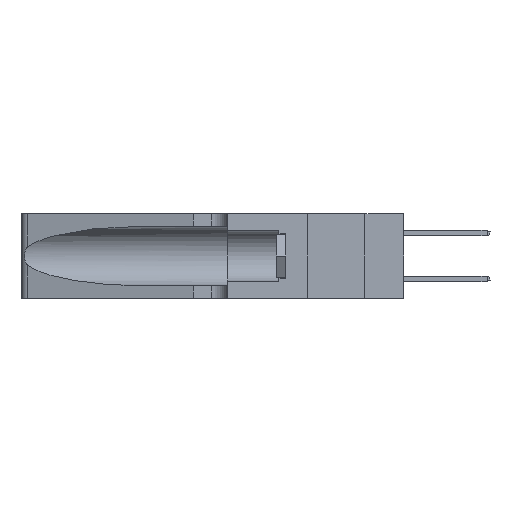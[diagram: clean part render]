
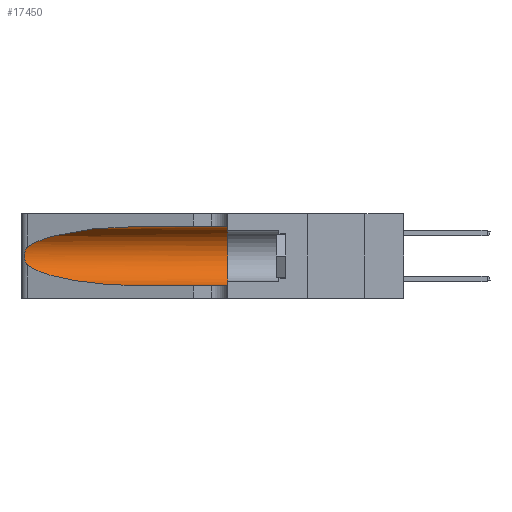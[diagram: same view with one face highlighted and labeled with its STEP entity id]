
A CAD part, left-side view. The second image highlights one B-rep face of the part: STEP entity #17450.
In plain terms, the highlighted cylindrical face has radius 3.308 mm (diameter 6.617 mm), a partial arc.
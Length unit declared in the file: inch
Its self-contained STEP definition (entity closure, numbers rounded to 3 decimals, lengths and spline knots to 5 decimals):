
#87 = CARTESIAN_POINT ( 'NONE',  ( 0.18966, 0.96281, 0.05475 ) ) ;
#588 = EDGE_CURVE ( 'NONE', #19616, #23437, #5162, .T. ) ;
#668 = CARTESIAN_POINT ( 'NONE',  ( 0.26075, 1.23896, 0.19203 ) ) ;
#1308 = CARTESIAN_POINT ( 'NONE',  ( 0.25639, 1.23186, 0.15144 ) ) ;
#2458 = CARTESIAN_POINT ( 'NONE',  ( 0.1305, 1.61858, 0.31525 ) ) ;
#2461 =( BOUNDED_CURVE ( )  B_SPLINE_CURVE ( 3, ( #14594, #11994, #22267, #20151 ),
 .UNSPECIFIED., .F., .T. ) 
 B_SPLINE_CURVE_WITH_KNOTS ( ( 4, 4 ),
 ( 1.5708, 2.84003 ),
 .UNSPECIFIED. ) 
 CURVE ( )  GEOMETRIC_REPRESENTATION_ITEM ( )  RATIONAL_B_SPLINE_CURVE ( ( 1., 0.87, 0.87, 1. ) ) 
 REPRESENTATION_ITEM ( '' )  );
#3308 = EDGE_CURVE ( 'NONE', #19616, #25562, #2461, .T. ) ;
#3708 = CARTESIAN_POINT ( 'NONE',  ( 0.1305, 0.72297, 0.05475 ) ) ;
#3767 = CARTESIAN_POINT ( 'NONE',  ( 0.25487, 1.22718, 0.22369 ) ) ;
#4150 = CARTESIAN_POINT ( 'NONE',  ( 0.1305, 0.35, 0.31525 ) ) ;
#5162 = LINE ( 'NONE', #2458, #22549 ) ;
#5173 = CARTESIAN_POINT ( 'NONE',  ( 0.25789, 1.23486, 0.15765 ) ) ;
#5747 = CARTESIAN_POINT ( 'NONE',  ( 0.25487, 1.22718, 0.14631 ) ) ;
#5825 = CARTESIAN_POINT ( 'NONE',  ( 0.26018, 1.23835, 0.19895 ) ) ;
#6298 = ORIENTED_EDGE ( 'NONE', *, *, #21303, .F. ) ;
#6315 = CARTESIAN_POINT ( 'NONE',  ( 0.25487, 1.22718, 0.22369 ) ) ;
#7749 = CARTESIAN_POINT ( 'NONE',  ( 0.1305, 1.61858, 0.185 ) ) ;
#7770 = CARTESIAN_POINT ( 'NONE',  ( 0.25639, 1.23184, 0.21858 ) ) ;
#8176 = EDGE_LOOP ( 'NONE', ( #15291, #21233, #22912, #13807, #6298, #23197 ) ) ;
#8428 = DIRECTION ( 'NONE',  ( 0., -1., 0. ) ) ;
#8626 = CARTESIAN_POINT ( 'NONE',  ( 0.26075, 1.23896, 0.178 ) ) ;
#9104 = CARTESIAN_POINT ( 'NONE',  ( 0.25854, 1.2359, 0.20912 ) ) ;
#9797 = VERTEX_POINT ( 'NONE', #15335 ) ;
#9818 = CARTESIAN_POINT ( 'NONE',  ( 0.2373, 1.15595, 0.08982 ) ) ;
#9870 = AXIS2_PLACEMENT_3D ( 'NONE', #19669, #17270, #13297 ) ;
#9951 = CIRCLE ( 'NONE', #9870, 0.13025 ) ;
#11065 = CARTESIAN_POINT ( 'NONE',  ( 0.25555, 1.22994, 0.2215 ) ) ;
#11994 = CARTESIAN_POINT ( 'NONE',  ( 0.18966, 0.96281, 0.31525 ) ) ;
#12639 = VERTEX_POINT ( 'NONE', #22845 ) ;
#13208 = CARTESIAN_POINT ( 'NONE',  ( 0.25856, 1.23593, 0.16098 ) ) ;
#13297 = DIRECTION ( 'NONE',  ( 0., 0., 1. ) ) ;
#13752 = DIRECTION ( 'NONE',  ( 0., 0., -1. ) ) ;
#13782 = CARTESIAN_POINT ( 'NONE',  ( 0.25787, 1.23484, 0.2124 ) ) ;
#13807 = ORIENTED_EDGE ( 'NONE', *, *, #19516, .T. ) ;
#13856 = VECTOR ( 'NONE', #8428, 39.37008 ) ;
#14523 = EDGE_CURVE ( 'NONE', #25562, #9797, #21310, .T. ) ;
#14594 = CARTESIAN_POINT ( 'NONE',  ( 0.1305, 0.72297, 0.31525 ) ) ;
#15291 = ORIENTED_EDGE ( 'NONE', *, *, #3308, .T. ) ;
#15335 = CARTESIAN_POINT ( 'NONE',  ( 0.25487, 1.22718, 0.14631 ) ) ;
#15519 = CARTESIAN_POINT ( 'NONE',  ( 0.25487, 1.22718, 0.14631 ) ) ;
#17270 = DIRECTION ( 'NONE',  ( 0., 1., 0. ) ) ;
#17450 = ADVANCED_FACE ( 'NONE', ( #18200 ), #18856, .F. ) ;
#18200 = FACE_OUTER_BOUND ( 'NONE', #8176, .T. ) ;
#18646 = DIRECTION ( 'NONE',  ( 0., -1., 0. ) ) ;
#18856 = CYLINDRICAL_SURFACE ( 'NONE', #24875, 0.13025 ) ;
#19297 = CARTESIAN_POINT ( 'NONE',  ( 0.1305, 1.61858, 0.05475 ) ) ;
#19516 = EDGE_CURVE ( 'NONE', #24859, #12639, #23667, .T. ) ;
#19616 = VERTEX_POINT ( 'NONE', #20596 ) ;
#19669 = CARTESIAN_POINT ( 'NONE',  ( 0.1305, 0.35, 0.185 ) ) ;
#20151 = CARTESIAN_POINT ( 'NONE',  ( 0.25487, 1.22718, 0.22369 ) ) ;
#20317 = CARTESIAN_POINT ( 'NONE',  ( 0.1305, 0.72297, 0.05475 ) ) ;
#20596 = CARTESIAN_POINT ( 'NONE',  ( 0.1305, 0.72297, 0.31525 ) ) ;
#21233 = ORIENTED_EDGE ( 'NONE', *, *, #14523, .T. ) ;
#21303 = EDGE_CURVE ( 'NONE', #23437, #12639, #9951, .T. ) ;
#21310 = B_SPLINE_CURVE_WITH_KNOTS ( 'NONE', 3,
 ( #6315, #11065, #7770, #13782, #9104, #5825, #668, #8626, #25427, #13208, #5173, #1308, #23568, #15519 ),
 .UNSPECIFIED., .F., .F.,
 ( 4, 2, 2, 2, 2, 2, 4 ),
 ( 0., 0.00027, 0.00053, 0.00107, 0.0016, 0.00187, 0.00214 ),
 .UNSPECIFIED. ) ;
#21721 = DIRECTION ( 'NONE',  ( 0., -1., 0. ) ) ;
#22234 = EDGE_CURVE ( 'NONE', #9797, #24859, #24049, .T. ) ;
#22267 = CARTESIAN_POINT ( 'NONE',  ( 0.2373, 1.15595, 0.28018 ) ) ;
#22549 = VECTOR ( 'NONE', #18646, 39.37008 ) ;
#22845 = CARTESIAN_POINT ( 'NONE',  ( 0.1305, 0.35, 0.05475 ) ) ;
#22912 = ORIENTED_EDGE ( 'NONE', *, *, #22234, .T. ) ;
#23197 = ORIENTED_EDGE ( 'NONE', *, *, #588, .F. ) ;
#23437 = VERTEX_POINT ( 'NONE', #4150 ) ;
#23568 = CARTESIAN_POINT ( 'NONE',  ( 0.25555, 1.22993, 0.14849 ) ) ;
#23667 = LINE ( 'NONE', #19297, #13856 ) ;
#24049 =( BOUNDED_CURVE ( )  B_SPLINE_CURVE ( 3, ( #5747, #9818, #87, #20317 ),
 .UNSPECIFIED., .F., .T. ) 
 B_SPLINE_CURVE_WITH_KNOTS ( ( 4, 4 ),
 ( 3.44316, 4.71239 ),
 .UNSPECIFIED. ) 
 CURVE ( )  GEOMETRIC_REPRESENTATION_ITEM ( )  RATIONAL_B_SPLINE_CURVE ( ( 1., 0.87, 0.87, 1. ) ) 
 REPRESENTATION_ITEM ( '' )  );
#24859 = VERTEX_POINT ( 'NONE', #3708 ) ;
#24875 = AXIS2_PLACEMENT_3D ( 'NONE', #7749, #21721, #13752 ) ;
#25427 = CARTESIAN_POINT ( 'NONE',  ( 0.26017, 1.23833, 0.17102 ) ) ;
#25562 = VERTEX_POINT ( 'NONE', #3767 ) ;
